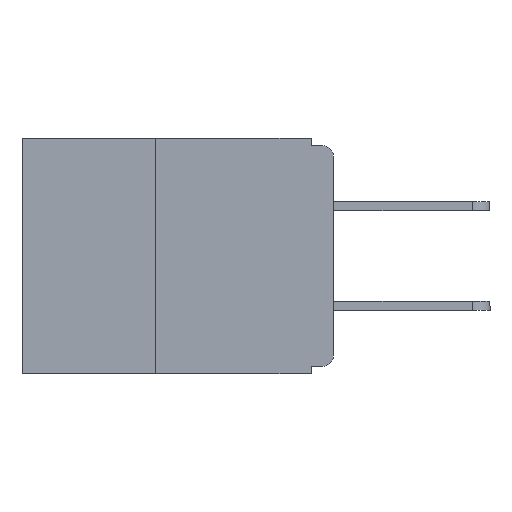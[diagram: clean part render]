
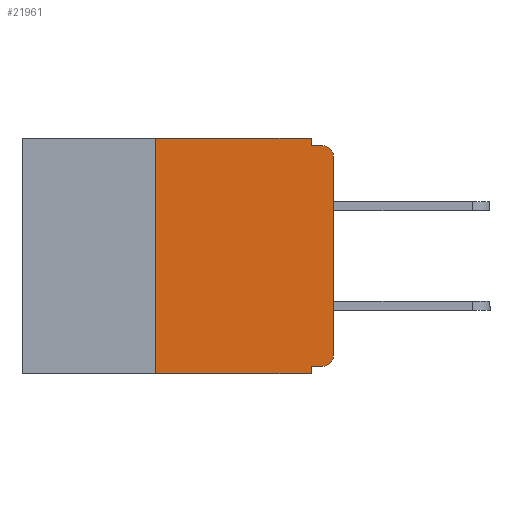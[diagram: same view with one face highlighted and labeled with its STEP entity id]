
A CAD part, left-side view. The second image highlights one B-rep face of the part: STEP entity #21961.
In plain terms, the highlighted planar face has unit normal (-1, 0, 0).
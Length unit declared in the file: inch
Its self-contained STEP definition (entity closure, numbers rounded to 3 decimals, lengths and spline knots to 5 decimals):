
#168 = VERTEX_POINT ( 'NONE', #970 ) ;
#179 = VERTEX_POINT ( 'NONE', #20166 ) ;
#588 = LINE ( 'NONE', #20920, #4348 ) ;
#970 = CARTESIAN_POINT ( 'NONE',  ( 0., 0.015, -0.32 ) ) ;
#1244 = LINE ( 'NONE', #1271, #10157 ) ;
#1271 = CARTESIAN_POINT ( 'NONE',  ( 0., 0.25, -0.33 ) ) ;
#1770 = LINE ( 'NONE', #4831, #19620 ) ;
#2067 = CARTESIAN_POINT ( 'NONE',  ( 0., 0., 0. ) ) ;
#2119 = DIRECTION ( 'NONE',  ( 0., 0., 1. ) ) ;
#2253 = EDGE_CURVE ( 'NONE', #8277, #9415, #1244, .T. ) ;
#2572 = CARTESIAN_POINT ( 'NONE',  ( 0., 0.25, 0. ) ) ;
#2763 = EDGE_CURVE ( 'NONE', #168, #179, #10133, .T. ) ;
#3027 = VECTOR ( 'NONE', #2119, 39.37008 ) ;
#3608 = DIRECTION ( 'NONE',  ( 0., -1., 0. ) ) ;
#3693 = LINE ( 'NONE', #3754, #16456 ) ;
#3754 = CARTESIAN_POINT ( 'NONE',  ( 0., 0.437, 0. ) ) ;
#4348 = VECTOR ( 'NONE', #20772, 39.37008 ) ;
#4784 = EDGE_CURVE ( 'NONE', #10331, #5454, #588, .T. ) ;
#4831 = CARTESIAN_POINT ( 'NONE',  ( 0., 0., -0.01 ) ) ;
#5207 = CARTESIAN_POINT ( 'NONE',  ( 0., 0.437, -0.33 ) ) ;
#5454 = VERTEX_POINT ( 'NONE', #11584 ) ;
#5911 = EDGE_CURVE ( 'NONE', #9415, #10331, #3693, .T. ) ;
#5997 = PLANE ( 'NONE',  #10010 ) ;
#6109 = AXIS2_PLACEMENT_3D ( 'NONE', #21241, #11487, #16725 ) ;
#6271 = VERTEX_POINT ( 'NONE', #13653 ) ;
#6355 = VECTOR ( 'NONE', #21779, 39.37008 ) ;
#7610 = EDGE_CURVE ( 'NONE', #6271, #10629, #11883, .T. ) ;
#7657 = ORIENTED_EDGE ( 'NONE', *, *, #2763, .T. ) ;
#7839 = DIRECTION ( 'NONE',  ( 1., 0., 0. ) ) ;
#7959 = DIRECTION ( 'NONE',  ( 0., 0., 1. ) ) ;
#8153 = DIRECTION ( 'NONE',  ( 0., 0., -1. ) ) ;
#8265 = DIRECTION ( 'NONE',  ( -1., 0., 0. ) ) ;
#8277 = VERTEX_POINT ( 'NONE', #17537 ) ;
#8359 = CARTESIAN_POINT ( 'NONE',  ( 0., 0.015, -0.025 ) ) ;
#9415 = VERTEX_POINT ( 'NONE', #2572 ) ;
#9463 = EDGE_CURVE ( 'NONE', #179, #6271, #16914, .T. ) ;
#9631 = VERTEX_POINT ( 'NONE', #21792 ) ;
#10010 = AXIS2_PLACEMENT_3D ( 'NONE', #18048, #7839, #19647 ) ;
#10133 = CIRCLE ( 'NONE', #6109, 0.015 ) ;
#10157 = VECTOR ( 'NONE', #7959, 39.37008 ) ;
#10270 = LINE ( 'NONE', #12818, #14353 ) ;
#10331 = VERTEX_POINT ( 'NONE', #20306 ) ;
#10629 = VERTEX_POINT ( 'NONE', #15118 ) ;
#11487 = DIRECTION ( 'NONE',  ( -1., 0., 0. ) ) ;
#11531 = LINE ( 'NONE', #11886, #6355 ) ;
#11584 = CARTESIAN_POINT ( 'NONE',  ( 0., 0.031, -0.01 ) ) ;
#11883 = CIRCLE ( 'NONE', #20849, 0.015 ) ;
#11886 = CARTESIAN_POINT ( 'NONE',  ( 0., 0.031, -0.33 ) ) ;
#12125 = VECTOR ( 'NONE', #22001, 39.37008 ) ;
#12580 = DIRECTION ( 'NONE',  ( 0., 1., 0. ) ) ;
#12656 = LINE ( 'NONE', #5207, #12125 ) ;
#12818 = CARTESIAN_POINT ( 'NONE',  ( 0., 0., -0.32 ) ) ;
#13198 = EDGE_LOOP ( 'NONE', ( #15432, #15560, #15027, #14855, #14642, #13840, #14063, #13633, #13240, #7657 ) ) ;
#13240 = ORIENTED_EDGE ( 'NONE', *, *, #13394, .F. ) ;
#13394 = EDGE_CURVE ( 'NONE', #168, #9631, #10270, .T. ) ;
#13633 = ORIENTED_EDGE ( 'NONE', *, *, #18957, .F. ) ;
#13653 = CARTESIAN_POINT ( 'NONE',  ( 0., 0., -0.025 ) ) ;
#13840 = ORIENTED_EDGE ( 'NONE', *, *, #2253, .F. ) ;
#14063 = ORIENTED_EDGE ( 'NONE', *, *, #21026, .T. ) ;
#14353 = VECTOR ( 'NONE', #12580, 39.37008 ) ;
#14642 = ORIENTED_EDGE ( 'NONE', *, *, #5911, .F. ) ;
#14819 = CARTESIAN_POINT ( 'NONE',  ( 0., 0.031, -0.33 ) ) ;
#14855 = ORIENTED_EDGE ( 'NONE', *, *, #4784, .F. ) ;
#15027 = ORIENTED_EDGE ( 'NONE', *, *, #22122, .F. ) ;
#15118 = CARTESIAN_POINT ( 'NONE',  ( 0., 0.015, -0.01 ) ) ;
#15432 = ORIENTED_EDGE ( 'NONE', *, *, #9463, .T. ) ;
#15560 = ORIENTED_EDGE ( 'NONE', *, *, #7610, .T. ) ;
#16456 = VECTOR ( 'NONE', #3608, 39.37008 ) ;
#16725 = DIRECTION ( 'NONE',  ( 0., 0., -1. ) ) ;
#16909 = DIRECTION ( 'NONE',  ( 0., -1., 0. ) ) ;
#16914 = LINE ( 'NONE', #2067, #3027 ) ;
#17537 = CARTESIAN_POINT ( 'NONE',  ( 0., 0.25, -0.33 ) ) ;
#18048 = CARTESIAN_POINT ( 'NONE',  ( 0., 0.437, 0. ) ) ;
#18776 = VERTEX_POINT ( 'NONE', #14819 ) ;
#18900 = FACE_OUTER_BOUND ( 'NONE', #13198, .T. ) ;
#18957 = EDGE_CURVE ( 'NONE', #9631, #18776, #11531, .T. ) ;
#19620 = VECTOR ( 'NONE', #16909, 39.37008 ) ;
#19647 = DIRECTION ( 'NONE',  ( 0., 0., -1. ) ) ;
#20166 = CARTESIAN_POINT ( 'NONE',  ( 0., 0., -0.305 ) ) ;
#20306 = CARTESIAN_POINT ( 'NONE',  ( 0., 0.031, 0. ) ) ;
#20772 = DIRECTION ( 'NONE',  ( 0., 0., -1. ) ) ;
#20849 = AXIS2_PLACEMENT_3D ( 'NONE', #8359, #8265, #8153 ) ;
#20920 = CARTESIAN_POINT ( 'NONE',  ( 0., 0.031, 0. ) ) ;
#21026 = EDGE_CURVE ( 'NONE', #8277, #18776, #12656, .T. ) ;
#21241 = CARTESIAN_POINT ( 'NONE',  ( 0., 0.015, -0.305 ) ) ;
#21779 = DIRECTION ( 'NONE',  ( 0., 0., -1. ) ) ;
#21792 = CARTESIAN_POINT ( 'NONE',  ( 0., 0.031, -0.32 ) ) ;
#21961 = ADVANCED_FACE ( 'NONE', ( #18900 ), #5997, .F. ) ;
#22001 = DIRECTION ( 'NONE',  ( 0., -1., 0. ) ) ;
#22122 = EDGE_CURVE ( 'NONE', #5454, #10629, #1770, .T. ) ;
